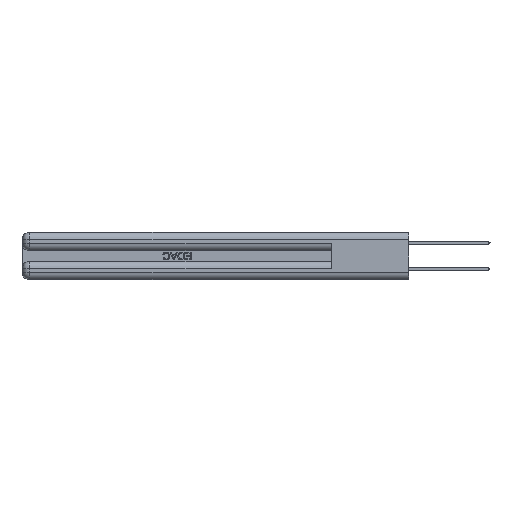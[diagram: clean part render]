
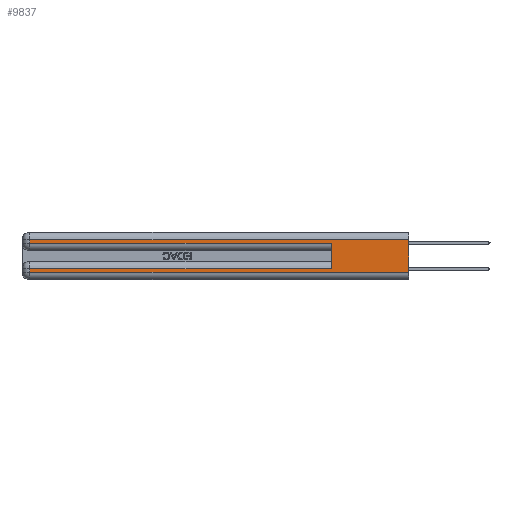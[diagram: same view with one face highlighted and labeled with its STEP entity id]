
A CAD part, left-side view. The second image highlights one B-rep face of the part: STEP entity #9837.
In plain terms, the highlighted planar face has unit normal (-1, 0, 0).
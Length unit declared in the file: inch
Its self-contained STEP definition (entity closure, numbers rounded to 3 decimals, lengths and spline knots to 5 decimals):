
#206 = LINE ( 'NONE', #44960, #37675 ) ;
#448 = VECTOR ( 'NONE', #22456, 39.37008 ) ;
#815 = DIRECTION ( 'NONE',  ( 0., 0., -1. ) ) ;
#1660 = LINE ( 'NONE', #49313, #448 ) ;
#1779 = VERTEX_POINT ( 'NONE', #12086 ) ;
#2215 = DIRECTION ( 'NONE',  ( 0., -1., 0. ) ) ;
#3540 = LINE ( 'NONE', #25406, #44557 ) ;
#5015 = DIRECTION ( 'NONE',  ( 0., 1., 0. ) ) ;
#5196 = ORIENTED_EDGE ( 'NONE', *, *, #13942, .T. ) ;
#5815 = LINE ( 'NONE', #45354, #44365 ) ;
#5961 = EDGE_CURVE ( 'NONE', #24155, #42950, #5815, .T. ) ;
#6008 = LINE ( 'NONE', #45848, #33150 ) ;
#6221 = ORIENTED_EDGE ( 'NONE', *, *, #5961, .F. ) ;
#6999 = DIRECTION ( 'NONE',  ( 0., 0., 1. ) ) ;
#9140 = CARTESIAN_POINT ( 'NONE',  ( 0., 2.94, 0.285 ) ) ;
#9837 = ADVANCED_FACE ( 'NONE', ( #30009 ), #46979, .F. ) ;
#10463 = DIRECTION ( 'NONE',  ( 0., 0., -1. ) ) ;
#12086 = CARTESIAN_POINT ( 'NONE',  ( 0., 2.94, 0.085 ) ) ;
#13942 = EDGE_CURVE ( 'NONE', #46199, #42950, #3540, .T. ) ;
#14218 = CARTESIAN_POINT ( 'NONE',  ( 0., 0.6, 0.285 ) ) ;
#14320 = CARTESIAN_POINT ( 'NONE',  ( 0., 0., 0.06 ) ) ;
#14833 = ORIENTED_EDGE ( 'NONE', *, *, #24007, .T. ) ;
#15987 = EDGE_CURVE ( 'NONE', #34613, #16189, #1660, .T. ) ;
#16189 = VERTEX_POINT ( 'NONE', #27521 ) ;
#18460 = ORIENTED_EDGE ( 'NONE', *, *, #25939, .T. ) ;
#18945 = DIRECTION ( 'NONE',  ( 0., 0., -1. ) ) ;
#19471 = AXIS2_PLACEMENT_3D ( 'NONE', #39301, #23996, #815 ) ;
#20992 = LINE ( 'NONE', #14320, #49218 ) ;
#21608 = DIRECTION ( 'NONE',  ( 0., 1., 0. ) ) ;
#22456 = DIRECTION ( 'NONE',  ( 0., 0., -1. ) ) ;
#22778 = LINE ( 'NONE', #24284, #30610 ) ;
#23424 = VECTOR ( 'NONE', #21608, 39.37008 ) ;
#23996 = DIRECTION ( 'NONE',  ( 1., 0., 0. ) ) ;
#24007 = EDGE_CURVE ( 'NONE', #34613, #38839, #43836, .T. ) ;
#24076 = EDGE_CURVE ( 'NONE', #46703, #16189, #20992, .T. ) ;
#24155 = VERTEX_POINT ( 'NONE', #34566 ) ;
#24284 = CARTESIAN_POINT ( 'NONE',  ( 0., 0., 0.085 ) ) ;
#24305 = EDGE_CURVE ( 'NONE', #24155, #1779, #22778, .T. ) ;
#25406 = CARTESIAN_POINT ( 'NONE',  ( 0., 0., 0.285 ) ) ;
#25494 = CARTESIAN_POINT ( 'NONE',  ( 0., 0., 0.31 ) ) ;
#25939 = EDGE_CURVE ( 'NONE', #38839, #46199, #206, .T. ) ;
#27338 = CARTESIAN_POINT ( 'NONE',  ( 0., 2.94, 0.06 ) ) ;
#27521 = CARTESIAN_POINT ( 'NONE',  ( 0., 0., 0.06 ) ) ;
#30009 = FACE_OUTER_BOUND ( 'NONE', #33048, .T. ) ;
#30610 = VECTOR ( 'NONE', #5015, 39.37008 ) ;
#30982 = ORIENTED_EDGE ( 'NONE', *, *, #24076, .T. ) ;
#33048 = EDGE_LOOP ( 'NONE', ( #47935, #14833, #18460, #5196, #6221, #38220, #34596, #30982 ) ) ;
#33150 = VECTOR ( 'NONE', #18945, 39.37008 ) ;
#34566 = CARTESIAN_POINT ( 'NONE',  ( 0., 0.6, 0.085 ) ) ;
#34596 = ORIENTED_EDGE ( 'NONE', *, *, #38664, .T. ) ;
#34613 = VERTEX_POINT ( 'NONE', #45758 ) ;
#37675 = VECTOR ( 'NONE', #10463, 39.37008 ) ;
#38220 = ORIENTED_EDGE ( 'NONE', *, *, #24305, .T. ) ;
#38664 = EDGE_CURVE ( 'NONE', #1779, #46703, #6008, .T. ) ;
#38839 = VERTEX_POINT ( 'NONE', #43640 ) ;
#39301 = CARTESIAN_POINT ( 'NONE',  ( 0., 0., 0.37 ) ) ;
#42950 = VERTEX_POINT ( 'NONE', #14218 ) ;
#43640 = CARTESIAN_POINT ( 'NONE',  ( 0., 2.94, 0.31 ) ) ;
#43836 = LINE ( 'NONE', #25494, #23424 ) ;
#44365 = VECTOR ( 'NONE', #6999, 39.37008 ) ;
#44557 = VECTOR ( 'NONE', #2215, 39.37008 ) ;
#44960 = CARTESIAN_POINT ( 'NONE',  ( 0., 2.94, 0.37 ) ) ;
#45115 = DIRECTION ( 'NONE',  ( 0., -1., 0. ) ) ;
#45354 = CARTESIAN_POINT ( 'NONE',  ( 0., 0.6, 0.145 ) ) ;
#45758 = CARTESIAN_POINT ( 'NONE',  ( 0., 0., 0.31 ) ) ;
#45848 = CARTESIAN_POINT ( 'NONE',  ( 0., 2.94, 0.37 ) ) ;
#46199 = VERTEX_POINT ( 'NONE', #9140 ) ;
#46703 = VERTEX_POINT ( 'NONE', #27338 ) ;
#46979 = PLANE ( 'NONE',  #19471 ) ;
#47935 = ORIENTED_EDGE ( 'NONE', *, *, #15987, .F. ) ;
#49218 = VECTOR ( 'NONE', #45115, 39.37008 ) ;
#49313 = CARTESIAN_POINT ( 'NONE',  ( 0., 0., 0.37 ) ) ;
